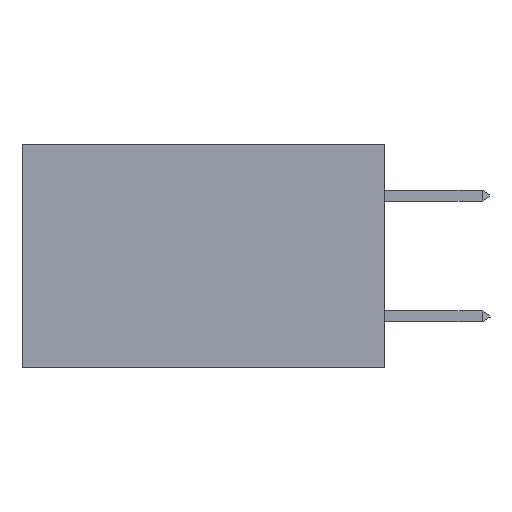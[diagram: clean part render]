
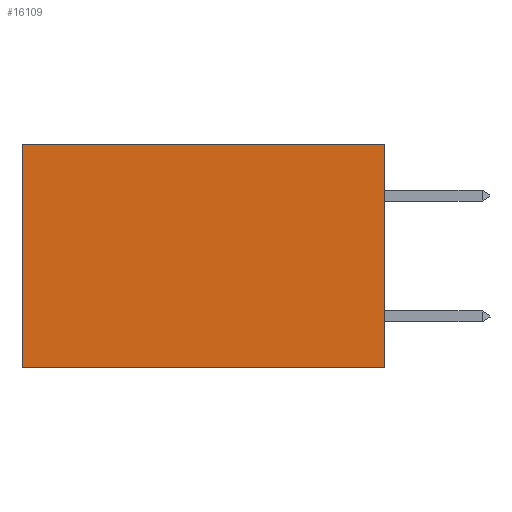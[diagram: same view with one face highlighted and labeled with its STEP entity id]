
A CAD part, left-side view. The second image highlights one B-rep face of the part: STEP entity #16109.
In plain terms, the highlighted planar face has unit normal (-1, 0, 0).
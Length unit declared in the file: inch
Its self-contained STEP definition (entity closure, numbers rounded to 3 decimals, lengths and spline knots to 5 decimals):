
#224 = CARTESIAN_POINT ( 'NONE',  ( 0.2875, 0., 0. ) ) ;
#544 = DIRECTION ( 'NONE',  ( 0., 0., -1. ) ) ;
#796 = VERTEX_POINT ( 'NONE', #224 ) ;
#3714 = FACE_OUTER_BOUND ( 'NONE', #14079, .T. ) ;
#3724 = EDGE_CURVE ( 'NONE', #21113, #19807, #12785, .T. ) ;
#4261 = VECTOR ( 'NONE', #544, 39.37008 ) ;
#5057 = EDGE_CURVE ( 'NONE', #796, #8720, #14319, .T. ) ;
#6786 = PLANE ( 'NONE',  #22152 ) ;
#7424 = ORIENTED_EDGE ( 'NONE', *, *, #13724, .F. ) ;
#7519 = EDGE_CURVE ( 'NONE', #796, #21113, #12406, .T. ) ;
#7531 = CARTESIAN_POINT ( 'NONE',  ( 0.2875, 0., 0. ) ) ;
#7933 = VECTOR ( 'NONE', #15168, 39.37008 ) ;
#8125 = VECTOR ( 'NONE', #19124, 39.37008 ) ;
#8316 = VECTOR ( 'NONE', #19182, 39.37008 ) ;
#8720 = VERTEX_POINT ( 'NONE', #21759 ) ;
#10208 = CARTESIAN_POINT ( 'NONE',  ( 0.2875, 0., 0. ) ) ;
#11139 = CARTESIAN_POINT ( 'NONE',  ( 0.2875, 0.6, 0. ) ) ;
#11896 = DIRECTION ( 'NONE',  ( 0., 0., -1. ) ) ;
#12406 = LINE ( 'NONE', #15094, #7933 ) ;
#12785 = LINE ( 'NONE', #17442, #8316 ) ;
#12919 = CARTESIAN_POINT ( 'NONE',  ( 0.2875, 0.6, -0.37 ) ) ;
#13110 = LINE ( 'NONE', #17386, #8125 ) ;
#13662 = ORIENTED_EDGE ( 'NONE', *, *, #5057, .F. ) ;
#13724 = EDGE_CURVE ( 'NONE', #8720, #19807, #13110, .T. ) ;
#14079 = EDGE_LOOP ( 'NONE', ( #22199, #7424, #13662, #21755 ) ) ;
#14319 = LINE ( 'NONE', #7531, #4261 ) ;
#15094 = CARTESIAN_POINT ( 'NONE',  ( 0.2875, 0., 0. ) ) ;
#15168 = DIRECTION ( 'NONE',  ( 0., 1., 0. ) ) ;
#16109 = ADVANCED_FACE ( 'NONE', ( #3714 ), #6786, .F. ) ;
#17386 = CARTESIAN_POINT ( 'NONE',  ( 0.2875, 0., -0.37 ) ) ;
#17442 = CARTESIAN_POINT ( 'NONE',  ( 0.2875, 0.6, 0. ) ) ;
#19124 = DIRECTION ( 'NONE',  ( 0., 1., 0. ) ) ;
#19182 = DIRECTION ( 'NONE',  ( 0., 0., -1. ) ) ;
#19807 = VERTEX_POINT ( 'NONE', #12919 ) ;
#21113 = VERTEX_POINT ( 'NONE', #11139 ) ;
#21755 = ORIENTED_EDGE ( 'NONE', *, *, #7519, .T. ) ;
#21759 = CARTESIAN_POINT ( 'NONE',  ( 0.2875, 0., -0.37 ) ) ;
#22152 = AXIS2_PLACEMENT_3D ( 'NONE', #10208, #22170, #11896 ) ;
#22170 = DIRECTION ( 'NONE',  ( 1., 0., 0. ) ) ;
#22199 = ORIENTED_EDGE ( 'NONE', *, *, #3724, .T. ) ;
